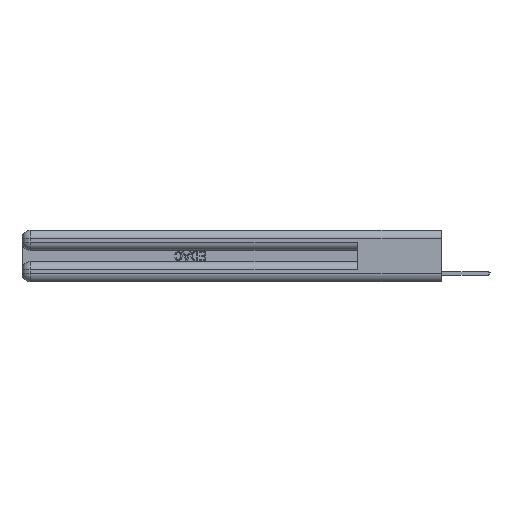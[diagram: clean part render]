
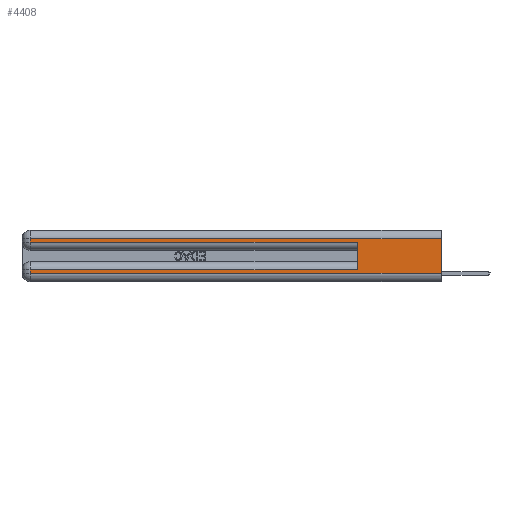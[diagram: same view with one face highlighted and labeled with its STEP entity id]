
A CAD part, left-side view. The second image highlights one B-rep face of the part: STEP entity #4408.
In plain terms, the highlighted planar face has unit normal (-1, 0, 0).
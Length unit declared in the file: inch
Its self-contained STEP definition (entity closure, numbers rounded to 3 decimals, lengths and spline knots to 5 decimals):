
#54 = VERTEX_POINT ( 'NONE', #20528 ) ;
#163 = EDGE_CURVE ( 'NONE', #54, #7049, #28681, .T. ) ;
#622 = DIRECTION ( 'NONE',  ( 0., 0., 1. ) ) ;
#1432 = DIRECTION ( 'NONE',  ( 0., 1., 0. ) ) ;
#1975 = AXIS2_PLACEMENT_3D ( 'NONE', #18455, #3304, #18347 ) ;
#2223 = CARTESIAN_POINT ( 'NONE',  ( 0., 0., 0.06 ) ) ;
#2719 = VERTEX_POINT ( 'NONE', #16194 ) ;
#2873 = LINE ( 'NONE', #20897, #21056 ) ;
#2956 = CARTESIAN_POINT ( 'NONE',  ( 0., 2.94, 0.37 ) ) ;
#3142 = CARTESIAN_POINT ( 'NONE',  ( 0., 0., 0.31 ) ) ;
#3304 = DIRECTION ( 'NONE',  ( 1., 0., 0. ) ) ;
#3823 = EDGE_CURVE ( 'NONE', #31006, #2719, #27363, .T. ) ;
#4145 = CARTESIAN_POINT ( 'NONE',  ( 0., 2.94, 0.06 ) ) ;
#4408 = ADVANCED_FACE ( 'NONE', ( #32481 ), #31201, .F. ) ;
#5028 = ORIENTED_EDGE ( 'NONE', *, *, #18362, .T. ) ;
#5397 = VECTOR ( 'NONE', #622, 39.37008 ) ;
#5442 = CARTESIAN_POINT ( 'NONE',  ( 0., 0., 0.285 ) ) ;
#5754 = DIRECTION ( 'NONE',  ( 0., 0., -1. ) ) ;
#6521 = CARTESIAN_POINT ( 'NONE',  ( 0., 0., 0.31 ) ) ;
#6772 = VECTOR ( 'NONE', #24723, 39.37008 ) ;
#6906 = VERTEX_POINT ( 'NONE', #27787 ) ;
#7049 = VERTEX_POINT ( 'NONE', #8158 ) ;
#7847 = DIRECTION ( 'NONE',  ( 0., -1., 0. ) ) ;
#7910 = CARTESIAN_POINT ( 'NONE',  ( 0., 0.6, 0.145 ) ) ;
#8158 = CARTESIAN_POINT ( 'NONE',  ( 0., 0.6, 0.285 ) ) ;
#8398 = ORIENTED_EDGE ( 'NONE', *, *, #14610, .T. ) ;
#8930 = VECTOR ( 'NONE', #18229, 39.37008 ) ;
#8968 = EDGE_CURVE ( 'NONE', #12627, #6906, #11718, .T. ) ;
#9948 = VECTOR ( 'NONE', #29980, 39.37008 ) ;
#10676 = EDGE_CURVE ( 'NONE', #12627, #2719, #2873, .T. ) ;
#11132 = LINE ( 'NONE', #12382, #9948 ) ;
#11413 = EDGE_CURVE ( 'NONE', #29510, #7049, #21411, .T. ) ;
#11718 = LINE ( 'NONE', #6521, #24331 ) ;
#12382 = CARTESIAN_POINT ( 'NONE',  ( 0., 2.94, 0.37 ) ) ;
#12627 = VERTEX_POINT ( 'NONE', #3142 ) ;
#13590 = ORIENTED_EDGE ( 'NONE', *, *, #8968, .T. ) ;
#13841 = VERTEX_POINT ( 'NONE', #15052 ) ;
#14610 = EDGE_CURVE ( 'NONE', #13841, #31006, #23941, .T. ) ;
#14714 = VECTOR ( 'NONE', #18483, 39.37008 ) ;
#15052 = CARTESIAN_POINT ( 'NONE',  ( 0., 2.94, 0.085 ) ) ;
#15522 = CARTESIAN_POINT ( 'NONE',  ( 0., 2.94, 0.285 ) ) ;
#16194 = CARTESIAN_POINT ( 'NONE',  ( 0., 0., 0.06 ) ) ;
#18229 = DIRECTION ( 'NONE',  ( 0., 0., -1. ) ) ;
#18347 = DIRECTION ( 'NONE',  ( 0., 0., -1. ) ) ;
#18362 = EDGE_CURVE ( 'NONE', #54, #13841, #20214, .T. ) ;
#18455 = CARTESIAN_POINT ( 'NONE',  ( 0., 0., 0.37 ) ) ;
#18483 = DIRECTION ( 'NONE',  ( 0., -1., 0. ) ) ;
#20214 = LINE ( 'NONE', #29677, #6772 ) ;
#20528 = CARTESIAN_POINT ( 'NONE',  ( 0., 0.6, 0.085 ) ) ;
#20897 = CARTESIAN_POINT ( 'NONE',  ( 0., 0., 0.37 ) ) ;
#21056 = VECTOR ( 'NONE', #5754, 39.37008 ) ;
#21411 = LINE ( 'NONE', #5442, #14714 ) ;
#21805 = ORIENTED_EDGE ( 'NONE', *, *, #10676, .F. ) ;
#23675 = ORIENTED_EDGE ( 'NONE', *, *, #163, .F. ) ;
#23941 = LINE ( 'NONE', #2956, #8930 ) ;
#24331 = VECTOR ( 'NONE', #1432, 39.37008 ) ;
#24723 = DIRECTION ( 'NONE',  ( 0., 1., 0. ) ) ;
#25682 = ORIENTED_EDGE ( 'NONE', *, *, #11413, .T. ) ;
#26126 = ORIENTED_EDGE ( 'NONE', *, *, #3823, .T. ) ;
#27363 = LINE ( 'NONE', #2223, #28574 ) ;
#27787 = CARTESIAN_POINT ( 'NONE',  ( 0., 2.94, 0.31 ) ) ;
#28060 = EDGE_LOOP ( 'NONE', ( #21805, #13590, #29552, #25682, #23675, #5028, #8398, #26126 ) ) ;
#28574 = VECTOR ( 'NONE', #7847, 39.37008 ) ;
#28681 = LINE ( 'NONE', #7910, #5397 ) ;
#29510 = VERTEX_POINT ( 'NONE', #15522 ) ;
#29552 = ORIENTED_EDGE ( 'NONE', *, *, #31838, .T. ) ;
#29677 = CARTESIAN_POINT ( 'NONE',  ( 0., 0., 0.085 ) ) ;
#29980 = DIRECTION ( 'NONE',  ( 0., 0., -1. ) ) ;
#31006 = VERTEX_POINT ( 'NONE', #4145 ) ;
#31201 = PLANE ( 'NONE',  #1975 ) ;
#31838 = EDGE_CURVE ( 'NONE', #6906, #29510, #11132, .T. ) ;
#32481 = FACE_OUTER_BOUND ( 'NONE', #28060, .T. ) ;
